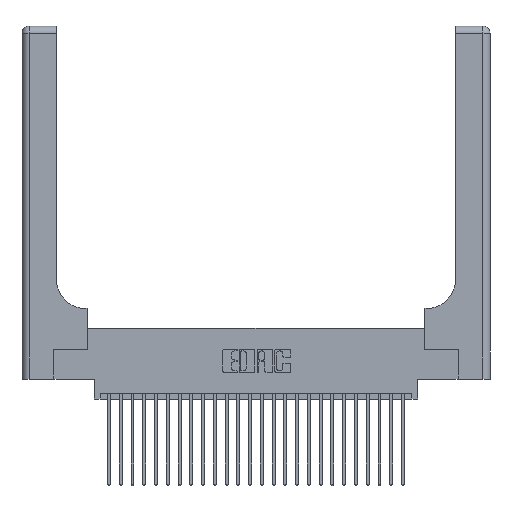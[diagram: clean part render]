
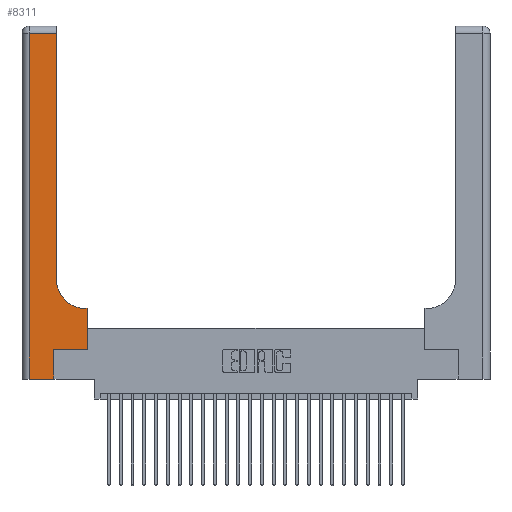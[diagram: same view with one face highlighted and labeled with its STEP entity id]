
A CAD part, top view. The second image highlights one B-rep face of the part: STEP entity #8311.
In plain terms, the highlighted planar face has unit normal (0, 0, 1).
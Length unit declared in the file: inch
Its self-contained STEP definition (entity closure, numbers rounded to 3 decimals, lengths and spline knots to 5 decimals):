
#481 = CARTESIAN_POINT ( 'NONE',  ( 0.269, 0., 0.37 ) ) ;
#1467 = LINE ( 'NONE', #2229, #19230 ) ;
#1767 = VERTEX_POINT ( 'NONE', #7549 ) ;
#2229 = CARTESIAN_POINT ( 'NONE',  ( 0.2915, 3., 0.37 ) ) ;
#3008 = EDGE_CURVE ( 'NONE', #6721, #1767, #1467, .T. ) ;
#3301 = VERTEX_POINT ( 'NONE', #19955 ) ;
#3543 = VERTEX_POINT ( 'NONE', #5776 ) ;
#3625 = AXIS2_PLACEMENT_3D ( 'NONE', #4020, #27741, #8084 ) ;
#3799 = EDGE_CURVE ( 'NONE', #6509, #3301, #6468, .T. ) ;
#4010 = LINE ( 'NONE', #10549, #24541 ) ;
#4020 = CARTESIAN_POINT ( 'NONE',  ( 0., 3., 0.37 ) ) ;
#4102 = DIRECTION ( 'NONE',  ( 0., 1., 0. ) ) ;
#4494 = ORIENTED_EDGE ( 'NONE', *, *, #3799, .T. ) ;
#4508 = CARTESIAN_POINT ( 'NONE',  ( 0.06, 2.94, 0.37 ) ) ;
#5593 = EDGE_CURVE ( 'NONE', #27531, #6509, #4010, .T. ) ;
#5776 = CARTESIAN_POINT ( 'NONE',  ( 0.5585, 0.25, 0.37 ) ) ;
#5835 = LINE ( 'NONE', #12014, #10537 ) ;
#6468 = LINE ( 'NONE', #481, #25651 ) ;
#6509 = VERTEX_POINT ( 'NONE', #22448 ) ;
#6721 = VERTEX_POINT ( 'NONE', #13055 ) ;
#6783 = VECTOR ( 'NONE', #16178, 39.37008 ) ;
#7549 = CARTESIAN_POINT ( 'NONE',  ( 0.2915, 2.94, 0.37 ) ) ;
#7665 = EDGE_CURVE ( 'NONE', #13763, #19855, #22495, .T. ) ;
#7759 = CARTESIAN_POINT ( 'NONE',  ( 0.2915, 0.6, 0.37 ) ) ;
#8023 = ORIENTED_EDGE ( 'NONE', *, *, #9564, .T. ) ;
#8084 = DIRECTION ( 'NONE',  ( -1., 0., 0. ) ) ;
#8311 = ADVANCED_FACE ( 'NONE', ( #18782 ), #12618, .F. ) ;
#9063 = CARTESIAN_POINT ( 'NONE',  ( 0.5415, 0.6, 0.37 ) ) ;
#9564 = EDGE_CURVE ( 'NONE', #3301, #3543, #19676, .T. ) ;
#10030 = ORIENTED_EDGE ( 'NONE', *, *, #5593, .T. ) ;
#10537 = VECTOR ( 'NONE', #14423, 39.37008 ) ;
#10549 = CARTESIAN_POINT ( 'NONE',  ( 0., 0., 0.37 ) ) ;
#10794 = ORIENTED_EDGE ( 'NONE', *, *, #7665, .T. ) ;
#10978 = VERTEX_POINT ( 'NONE', #4508 ) ;
#11040 = DIRECTION ( 'NONE',  ( 0., 0., -1. ) ) ;
#11140 = DIRECTION ( 'NONE',  ( 1., 0., 0. ) ) ;
#12014 = CARTESIAN_POINT ( 'NONE',  ( 0., 2.94, 0.37 ) ) ;
#12090 = DIRECTION ( 'NONE',  ( -1., 0., 0. ) ) ;
#12618 = PLANE ( 'NONE',  #3625 ) ;
#13055 = CARTESIAN_POINT ( 'NONE',  ( 0.2915, 0.85, 0.37 ) ) ;
#13567 = DIRECTION ( 'NONE',  ( 0., 1., 0. ) ) ;
#13744 = CARTESIAN_POINT ( 'NONE',  ( 0.5585, 0.6, 0.37 ) ) ;
#13763 = VERTEX_POINT ( 'NONE', #13744 ) ;
#14008 = VECTOR ( 'NONE', #15345, 39.37008 ) ;
#14423 = DIRECTION ( 'NONE',  ( -1., 0., 0. ) ) ;
#15345 = DIRECTION ( 'NONE',  ( 1., 0., 0. ) ) ;
#15970 = EDGE_CURVE ( 'NONE', #19855, #6721, #19974, .T. ) ;
#16178 = DIRECTION ( 'NONE',  ( 0., -1., 0. ) ) ;
#16455 = VECTOR ( 'NONE', #12090, 39.37008 ) ;
#16803 = VECTOR ( 'NONE', #26987, 39.37008 ) ;
#17480 = CARTESIAN_POINT ( 'NONE',  ( 0.5585, 0.25, 0.37 ) ) ;
#18782 = FACE_OUTER_BOUND ( 'NONE', #20198, .T. ) ;
#18968 = EDGE_CURVE ( 'NONE', #3543, #13763, #19818, .T. ) ;
#19036 = ORIENTED_EDGE ( 'NONE', *, *, #23978, .T. ) ;
#19230 = VECTOR ( 'NONE', #4102, 39.37008 ) ;
#19676 = LINE ( 'NONE', #21929, #14008 ) ;
#19818 = LINE ( 'NONE', #17480, #16803 ) ;
#19855 = VERTEX_POINT ( 'NONE', #9063 ) ;
#19955 = CARTESIAN_POINT ( 'NONE',  ( 0.269, 0.25, 0.37 ) ) ;
#19974 = CIRCLE ( 'NONE', #20468, 0.25 ) ;
#20198 = EDGE_LOOP ( 'NONE', ( #23715, #19036, #27076, #10030, #4494, #8023, #25603, #10794, #24243 ) ) ;
#20468 = AXIS2_PLACEMENT_3D ( 'NONE', #23989, #11040, #11140 ) ;
#21929 = CARTESIAN_POINT ( 'NONE',  ( 0.269, 0.25, 0.37 ) ) ;
#22448 = CARTESIAN_POINT ( 'NONE',  ( 0.269, 0., 0.37 ) ) ;
#22495 = LINE ( 'NONE', #7759, #16455 ) ;
#23399 = DIRECTION ( 'NONE',  ( 1., 0., 0. ) ) ;
#23596 = LINE ( 'NONE', #27022, #6783 ) ;
#23715 = ORIENTED_EDGE ( 'NONE', *, *, #3008, .T. ) ;
#23972 = CARTESIAN_POINT ( 'NONE',  ( 0.06, 0., 0.37 ) ) ;
#23978 = EDGE_CURVE ( 'NONE', #1767, #10978, #5835, .T. ) ;
#23989 = CARTESIAN_POINT ( 'NONE',  ( 0.5415, 0.85, 0.37 ) ) ;
#24243 = ORIENTED_EDGE ( 'NONE', *, *, #15970, .T. ) ;
#24541 = VECTOR ( 'NONE', #23399, 39.37008 ) ;
#25603 = ORIENTED_EDGE ( 'NONE', *, *, #18968, .T. ) ;
#25651 = VECTOR ( 'NONE', #13567, 39.37008 ) ;
#26564 = EDGE_CURVE ( 'NONE', #10978, #27531, #23596, .T. ) ;
#26987 = DIRECTION ( 'NONE',  ( 0., 1., 0. ) ) ;
#27022 = CARTESIAN_POINT ( 'NONE',  ( 0.06, 3., 0.37 ) ) ;
#27076 = ORIENTED_EDGE ( 'NONE', *, *, #26564, .T. ) ;
#27531 = VERTEX_POINT ( 'NONE', #23972 ) ;
#27741 = DIRECTION ( 'NONE',  ( 0., 0., -1. ) ) ;
